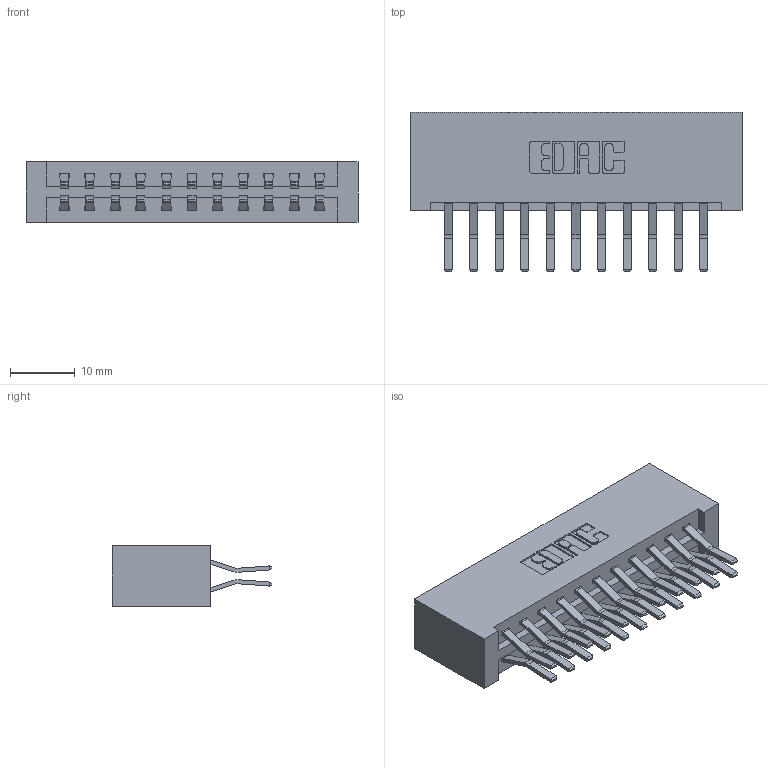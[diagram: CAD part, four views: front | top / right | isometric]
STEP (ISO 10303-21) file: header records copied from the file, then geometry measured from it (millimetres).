
FILE_DESCRIPTION (( 'STEP AP203' ), '1' );
FILE_NAME ('337-022-560-201.STEP', '2019-10-08T15:04:52', ( '' ), ( '' ), 'SwSTEP 2.0', 'SolidWorks 2016', '' );
FILE_SCHEMA (( 'CONFIG_CONTROL_DESIGN' ));
Length unit declared in the file: inch
Products named in the file (3): 345-292-001_560 Tail; 337 Part_No Mounting Lugs; 337-022-560-201
Assembly tree (23 placements, depth 2):
  337-022-560-201
    337 Part_No Mounting Lugs
    345-292-001_560 Tail  x22
Bounding box: 51.46 x 24.78 x 9.4 mm (x, y, z)
Volume: 5915.6 mm3; surface area: 6859.9 mm2
Topology: 23 solids, 23 shells, 1338 faces, 3961 edges, 2610 vertices
Faces by surface type: plane 902, cylinder 436
Entity records: 12349 total; most frequent: CARTESIAN_POINT 2106, ORIENTED_EDGE 2042, DIRECTION 1845, EDGE_CURVE 1021, VECTOR 897, LINE 897, VERTEX_POINT 678, AXIS2_PLACEMENT_3D 474
